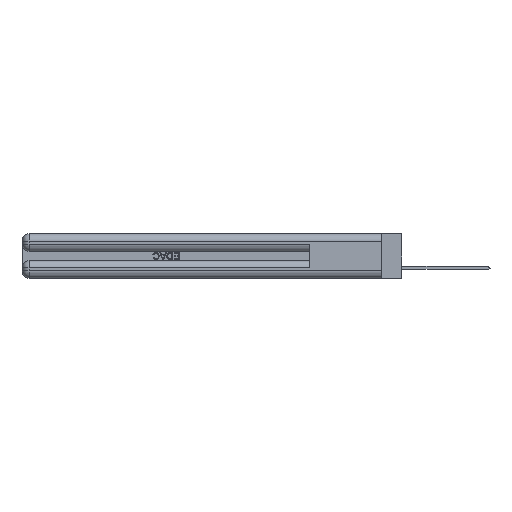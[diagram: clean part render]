
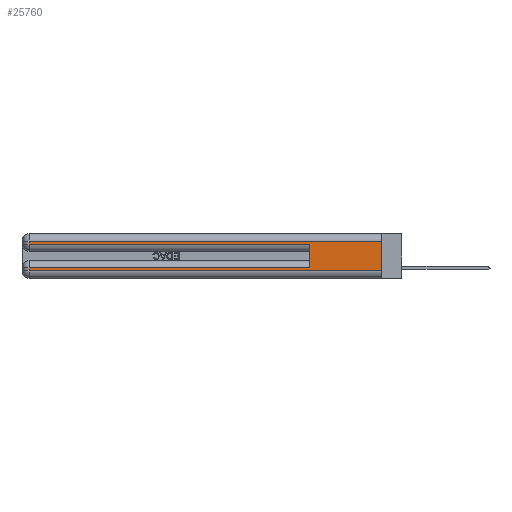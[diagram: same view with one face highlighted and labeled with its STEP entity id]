
A CAD part, left-side view. The second image highlights one B-rep face of the part: STEP entity #25760.
In plain terms, the highlighted planar face has unit normal (-1, 0, 0).
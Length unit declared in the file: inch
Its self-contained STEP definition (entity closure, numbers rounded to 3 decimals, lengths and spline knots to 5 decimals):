
#520 = DIRECTION ( 'NONE',  ( 0., 0., 1. ) ) ;
#629 = ORIENTED_EDGE ( 'NONE', *, *, #27899, .T. ) ;
#1157 = PLANE ( 'NONE',  #28220 ) ;
#1172 = ORIENTED_EDGE ( 'NONE', *, *, #34723, .T. ) ;
#1366 = DIRECTION ( 'NONE',  ( 0., 1., 0. ) ) ;
#1979 = EDGE_CURVE ( 'NONE', #3870, #8888, #14301, .T. ) ;
#2633 = CARTESIAN_POINT ( 'NONE',  ( 0., 2.94, 0.285 ) ) ;
#3312 = EDGE_CURVE ( 'NONE', #4235, #34185, #18761, .T. ) ;
#3426 = CARTESIAN_POINT ( 'NONE',  ( 0., 2.94, 0.31 ) ) ;
#3870 = VERTEX_POINT ( 'NONE', #31110 ) ;
#3896 = CARTESIAN_POINT ( 'NONE',  ( 0., 2.94, 0.37 ) ) ;
#4235 = VERTEX_POINT ( 'NONE', #3426 ) ;
#4581 = EDGE_LOOP ( 'NONE', ( #10313, #45428, #22671, #629, #10710, #29990, #11353, #1172 ) ) ;
#4622 = VERTEX_POINT ( 'NONE', #13296 ) ;
#4725 = CARTESIAN_POINT ( 'NONE',  ( 0., 0., 0.37 ) ) ;
#8888 = VERTEX_POINT ( 'NONE', #21648 ) ;
#10313 = ORIENTED_EDGE ( 'NONE', *, *, #37164, .F. ) ;
#10710 = ORIENTED_EDGE ( 'NONE', *, *, #24504, .F. ) ;
#11353 = ORIENTED_EDGE ( 'NONE', *, *, #1979, .T. ) ;
#11853 = LINE ( 'NONE', #34048, #31014 ) ;
#12485 = EDGE_CURVE ( 'NONE', #14632, #3870, #38267, .T. ) ;
#13296 = CARTESIAN_POINT ( 'NONE',  ( 0., 0.6, 0.285 ) ) ;
#14301 = LINE ( 'NONE', #3896, #34597 ) ;
#14632 = VERTEX_POINT ( 'NONE', #40202 ) ;
#14760 = VECTOR ( 'NONE', #42392, 39.37008 ) ;
#16177 = CARTESIAN_POINT ( 'NONE',  ( 0., 0., 0.31 ) ) ;
#16569 = VERTEX_POINT ( 'NONE', #39312 ) ;
#17015 = VECTOR ( 'NONE', #28497, 39.37008 ) ;
#17876 = LINE ( 'NONE', #30519, #40501 ) ;
#18404 = LINE ( 'NONE', #16177, #46907 ) ;
#18761 = LINE ( 'NONE', #45971, #14760 ) ;
#20730 = CARTESIAN_POINT ( 'NONE',  ( 0., 0., 0.31 ) ) ;
#20843 = VECTOR ( 'NONE', #1366, 39.37008 ) ;
#20914 = VECTOR ( 'NONE', #520, 39.37008 ) ;
#21648 = CARTESIAN_POINT ( 'NONE',  ( 0., 2.94, 0.06 ) ) ;
#21988 = DIRECTION ( 'NONE',  ( 0., 0., -1. ) ) ;
#22671 = ORIENTED_EDGE ( 'NONE', *, *, #3312, .T. ) ;
#23135 = DIRECTION ( 'NONE',  ( 0., 0., -1. ) ) ;
#24504 = EDGE_CURVE ( 'NONE', #14632, #4622, #26097, .T. ) ;
#25760 = ADVANCED_FACE ( 'NONE', ( #39399 ), #1157, .F. ) ;
#26097 = LINE ( 'NONE', #29692, #20914 ) ;
#27067 = DIRECTION ( 'NONE',  ( 0., -1., 0. ) ) ;
#27899 = EDGE_CURVE ( 'NONE', #34185, #4622, #11853, .T. ) ;
#28220 = AXIS2_PLACEMENT_3D ( 'NONE', #4725, #30594, #23135 ) ;
#28497 = DIRECTION ( 'NONE',  ( 0., -1., 0. ) ) ;
#28612 = LINE ( 'NONE', #47044, #17015 ) ;
#29692 = CARTESIAN_POINT ( 'NONE',  ( 0., 0.6, 0.145 ) ) ;
#29990 = ORIENTED_EDGE ( 'NONE', *, *, #12485, .T. ) ;
#30519 = CARTESIAN_POINT ( 'NONE',  ( 0., 0., 0.37 ) ) ;
#30594 = DIRECTION ( 'NONE',  ( 1., 0., 0. ) ) ;
#31014 = VECTOR ( 'NONE', #27067, 39.37008 ) ;
#31110 = CARTESIAN_POINT ( 'NONE',  ( 0., 2.94, 0.085 ) ) ;
#33574 = VERTEX_POINT ( 'NONE', #20730 ) ;
#34048 = CARTESIAN_POINT ( 'NONE',  ( 0., 0., 0.285 ) ) ;
#34185 = VERTEX_POINT ( 'NONE', #2633 ) ;
#34537 = CARTESIAN_POINT ( 'NONE',  ( 0., 0., 0.085 ) ) ;
#34597 = VECTOR ( 'NONE', #21988, 39.37008 ) ;
#34723 = EDGE_CURVE ( 'NONE', #8888, #16569, #28612, .T. ) ;
#37164 = EDGE_CURVE ( 'NONE', #33574, #16569, #17876, .T. ) ;
#38267 = LINE ( 'NONE', #34537, #20843 ) ;
#38559 = DIRECTION ( 'NONE',  ( 0., 1., 0. ) ) ;
#39312 = CARTESIAN_POINT ( 'NONE',  ( 0., 0., 0.06 ) ) ;
#39399 = FACE_OUTER_BOUND ( 'NONE', #4581, .T. ) ;
#40202 = CARTESIAN_POINT ( 'NONE',  ( 0., 0.6, 0.085 ) ) ;
#40501 = VECTOR ( 'NONE', #41891, 39.37008 ) ;
#41891 = DIRECTION ( 'NONE',  ( 0., 0., -1. ) ) ;
#42392 = DIRECTION ( 'NONE',  ( 0., 0., -1. ) ) ;
#43999 = EDGE_CURVE ( 'NONE', #33574, #4235, #18404, .T. ) ;
#45428 = ORIENTED_EDGE ( 'NONE', *, *, #43999, .T. ) ;
#45971 = CARTESIAN_POINT ( 'NONE',  ( 0., 2.94, 0.37 ) ) ;
#46907 = VECTOR ( 'NONE', #38559, 39.37008 ) ;
#47044 = CARTESIAN_POINT ( 'NONE',  ( 0., 0., 0.06 ) ) ;
